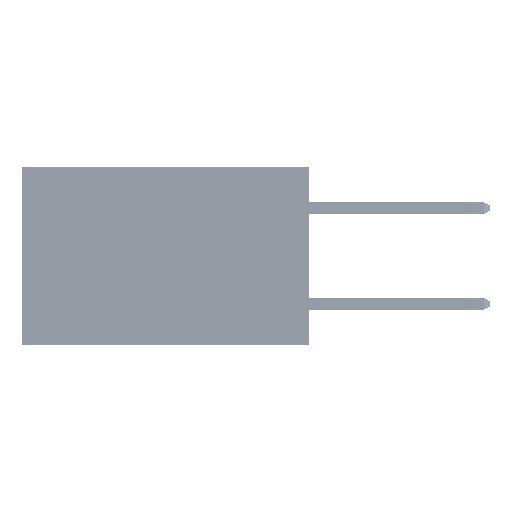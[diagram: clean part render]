
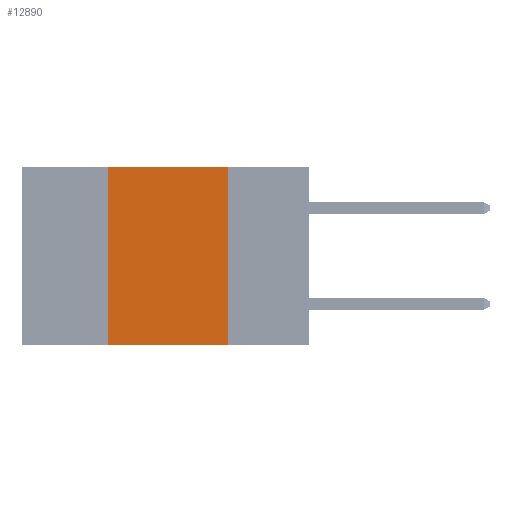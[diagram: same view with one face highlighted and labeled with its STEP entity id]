
A CAD part, left-side view. The second image highlights one B-rep face of the part: STEP entity #12890.
In plain terms, the highlighted planar face has unit normal (-1, 0, 0).
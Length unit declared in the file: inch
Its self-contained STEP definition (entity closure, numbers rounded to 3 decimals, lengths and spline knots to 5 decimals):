
#1638 = VECTOR ( 'NONE', #2504, 39.37008 ) ;
#2075 = EDGE_CURVE ( 'NONE', #17351, #16334, #24902, .T. ) ;
#2211 = EDGE_CURVE ( 'NONE', #17351, #42499, #18431, .T. ) ;
#2504 = DIRECTION ( 'NONE',  ( 0., 0., 1. ) ) ;
#2541 = VERTEX_POINT ( 'NONE', #17376 ) ;
#2811 = ORIENTED_EDGE ( 'NONE', *, *, #26003, .F. ) ;
#3324 = CARTESIAN_POINT ( 'NONE',  ( 0., 0.42, -0.37 ) ) ;
#3665 = ORIENTED_EDGE ( 'NONE', *, *, #2075, .F. ) ;
#4974 = CARTESIAN_POINT ( 'NONE',  ( 0., 0.42, 0. ) ) ;
#5750 = ORIENTED_EDGE ( 'NONE', *, *, #12405, .F. ) ;
#6736 = CARTESIAN_POINT ( 'NONE',  ( 0., 0.42, 0. ) ) ;
#7255 = CARTESIAN_POINT ( 'NONE',  ( 0., 0.6, 0. ) ) ;
#7549 = CARTESIAN_POINT ( 'NONE',  ( 0., 0.17, -0.37 ) ) ;
#10620 = DIRECTION ( 'NONE',  ( 0., 0., -1. ) ) ;
#10822 = PLANE ( 'NONE',  #24921 ) ;
#11853 = VECTOR ( 'NONE', #37365, 39.37008 ) ;
#12405 = EDGE_CURVE ( 'NONE', #2541, #42499, #25552, .T. ) ;
#12890 = ADVANCED_FACE ( 'NONE', ( #44913 ), #10822, .F. ) ;
#15447 = CARTESIAN_POINT ( 'NONE',  ( 0., 0.6, -0.37 ) ) ;
#15743 = ORIENTED_EDGE ( 'NONE', *, *, #2211, .T. ) ;
#16334 = VERTEX_POINT ( 'NONE', #4974 ) ;
#17351 = VERTEX_POINT ( 'NONE', #3324 ) ;
#17376 = CARTESIAN_POINT ( 'NONE',  ( 0., 0.17, 0. ) ) ;
#18027 = DIRECTION ( 'NONE',  ( 1., 0., 0. ) ) ;
#18431 = LINE ( 'NONE', #15447, #22311 ) ;
#19183 = DIRECTION ( 'NONE',  ( 0., -1., 0. ) ) ;
#22255 = CARTESIAN_POINT ( 'NONE',  ( 0., 0.6, 0. ) ) ;
#22311 = VECTOR ( 'NONE', #19183, 39.37008 ) ;
#24902 = LINE ( 'NONE', #6736, #1638 ) ;
#24921 = AXIS2_PLACEMENT_3D ( 'NONE', #22255, #18027, #33208 ) ;
#25552 = LINE ( 'NONE', #40743, #44768 ) ;
#26003 = EDGE_CURVE ( 'NONE', #16334, #2541, #41097, .T. ) ;
#30203 = EDGE_LOOP ( 'NONE', ( #5750, #2811, #3665, #15743 ) ) ;
#33208 = DIRECTION ( 'NONE',  ( 0., 0., -1. ) ) ;
#37365 = DIRECTION ( 'NONE',  ( 0., -1., 0. ) ) ;
#40743 = CARTESIAN_POINT ( 'NONE',  ( 0., 0.17, 0. ) ) ;
#41097 = LINE ( 'NONE', #7255, #11853 ) ;
#42499 = VERTEX_POINT ( 'NONE', #7549 ) ;
#44768 = VECTOR ( 'NONE', #10620, 39.37008 ) ;
#44913 = FACE_OUTER_BOUND ( 'NONE', #30203, .T. ) ;
